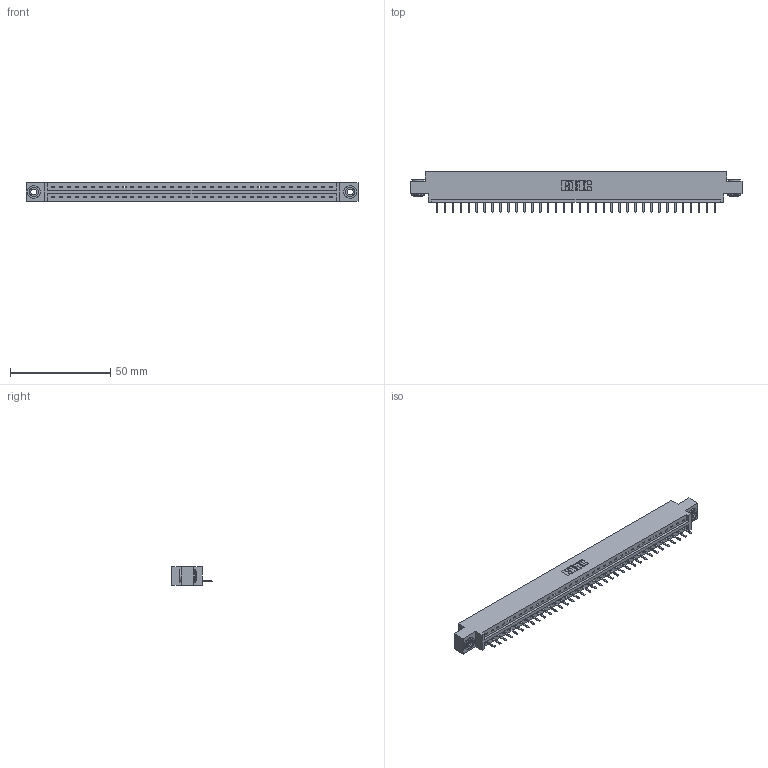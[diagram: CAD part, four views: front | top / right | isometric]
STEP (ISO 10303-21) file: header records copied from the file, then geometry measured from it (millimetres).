
FILE_DESCRIPTION (( 'STEP AP203' ), '1' );
FILE_NAME ('387-036-520-603.STEP', '2019-10-04T12:54:20', ( '' ), ( '' ), 'SwSTEP 2.0', 'SolidWorks 2016', '' );
FILE_SCHEMA (( 'CONFIG_CONTROL_DESIGN' ));
Length unit declared in the file: inch
Products named in the file (4): 387-036-520-603; 337 Part_0.170 Offset - 0.156 Dia-TH; 345-292-001_345-293-120; 345-250-002_345-250-002-102
Assembly tree (39 placements, depth 2):
  387-036-520-603
    337 Part_0.170 Offset - 0.156 Dia-TH
    345-292-001_345-293-120  x36
    345-250-002_345-250-002-102  x2
Bounding box: 165.66 x 20.02 x 9.4 mm (x, y, z)
Volume: 16940.7 mm3; surface area: 17428.8 mm2
Topology: 39 solids, 39 shells, 2532 faces, 7455 edges, 4870 vertices
Faces by surface type: plane 1812, cylinder 712, cone 8
Entity records: 28432 total; most frequent: CARTESIAN_POINT 4941, ORIENTED_EDGE 4894, DIRECTION 4193, EDGE_CURVE 2447, LINE 2291, VECTOR 2291, VERTEX_POINT 1626, AXIS2_PLACEMENT_3D 951
